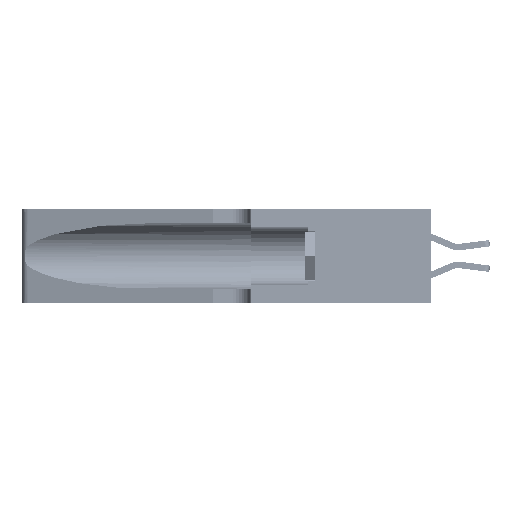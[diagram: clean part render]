
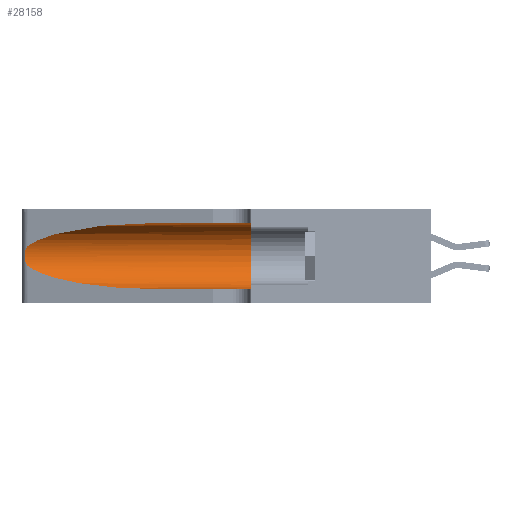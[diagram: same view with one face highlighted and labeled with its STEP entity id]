
A CAD part, left-side view. The second image highlights one B-rep face of the part: STEP entity #28158.
In plain terms, the highlighted cylindrical face has radius 3.308 mm (diameter 6.617 mm), a partial arc.
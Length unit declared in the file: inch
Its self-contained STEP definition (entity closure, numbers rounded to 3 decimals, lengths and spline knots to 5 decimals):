
#955 = EDGE_CURVE ( 'NONE', #9672, #32632, #32036, .T. ) ;
#1538 = DIRECTION ( 'NONE',  ( 0., -1., 0. ) ) ;
#1852 = DIRECTION ( 'NONE',  ( 0., 1., 0. ) ) ;
#2237 = ORIENTED_EDGE ( 'NONE', *, *, #9821, .T. ) ;
#2737 = CARTESIAN_POINT ( 'NONE',  ( 0.25487, 1.22718, 0.22369 ) ) ;
#3219 = CARTESIAN_POINT ( 'NONE',  ( 0.1305, 0.72297, 0.05475 ) ) ;
#3648 = VECTOR ( 'NONE', #16334, 39.37008 ) ;
#4323 = CARTESIAN_POINT ( 'NONE',  ( 0.25487, 1.22718, 0.22369 ) ) ;
#4564 = DIRECTION ( 'NONE',  ( 0., 0., -1. ) ) ;
#4665 = CIRCLE ( 'NONE', #30222, 0.13025 ) ;
#6470 = VERTEX_POINT ( 'NONE', #3219 ) ;
#8814 = CARTESIAN_POINT ( 'NONE',  ( 0.25639, 1.23184, 0.21858 ) ) ;
#9280 = EDGE_CURVE ( 'NONE', #32632, #34541, #4665, .T. ) ;
#9672 = VERTEX_POINT ( 'NONE', #33567 ) ;
#9786 = FACE_OUTER_BOUND ( 'NONE', #30155, .T. ) ;
#9821 = EDGE_CURVE ( 'NONE', #9672, #14651, #11032, .T. ) ;
#10964 = CARTESIAN_POINT ( 'NONE',  ( 0.25789, 1.23486, 0.15765 ) ) ;
#11032 =( BOUNDED_CURVE ( )  B_SPLINE_CURVE ( 3, ( #16282, #19307, #22348, #4323 ),
 .UNSPECIFIED., .F., .F. ) 
 B_SPLINE_CURVE_WITH_KNOTS ( ( 4, 4 ),
 ( 1.5708, 2.84003 ),
 .UNSPECIFIED. ) 
 CURVE ( )  GEOMETRIC_REPRESENTATION_ITEM ( )  RATIONAL_B_SPLINE_CURVE ( ( 1., 0.87, 0.87, 1. ) ) 
 REPRESENTATION_ITEM ( '' )  );
#11691 = CARTESIAN_POINT ( 'NONE',  ( 0.25555, 1.22994, 0.2215 ) ) ;
#11820 = CARTESIAN_POINT ( 'NONE',  ( 0.25854, 1.2359, 0.20912 ) ) ;
#11957 = CARTESIAN_POINT ( 'NONE',  ( 0.2373, 1.15595, 0.08982 ) ) ;
#13049 = EDGE_CURVE ( 'NONE', #14651, #28102, #31943, .T. ) ;
#13907 =( BOUNDED_CURVE ( )  B_SPLINE_CURVE ( 3, ( #14707, #11957, #18015, #24111 ),
 .UNSPECIFIED., .F., .F. ) 
 B_SPLINE_CURVE_WITH_KNOTS ( ( 4, 4 ),
 ( 3.44316, 4.71239 ),
 .UNSPECIFIED. ) 
 CURVE ( )  GEOMETRIC_REPRESENTATION_ITEM ( )  RATIONAL_B_SPLINE_CURVE ( ( 1., 0.87, 0.87, 1. ) ) 
 REPRESENTATION_ITEM ( '' )  );
#13972 = CARTESIAN_POINT ( 'NONE',  ( 0.25555, 1.22993, 0.14849 ) ) ;
#14651 = VERTEX_POINT ( 'NONE', #38706 ) ;
#14707 = CARTESIAN_POINT ( 'NONE',  ( 0.25487, 1.22718, 0.14631 ) ) ;
#14832 = CARTESIAN_POINT ( 'NONE',  ( 0.26075, 1.23896, 0.19203 ) ) ;
#15405 = ORIENTED_EDGE ( 'NONE', *, *, #35889, .T. ) ;
#16178 = CARTESIAN_POINT ( 'NONE',  ( 0.1305, 1.61858, 0.31525 ) ) ;
#16282 = CARTESIAN_POINT ( 'NONE',  ( 0.1305, 0.72297, 0.31525 ) ) ;
#16334 = DIRECTION ( 'NONE',  ( 0., -1., 0. ) ) ;
#16691 = CARTESIAN_POINT ( 'NONE',  ( 0.1305, 0.35, 0.05475 ) ) ;
#17156 = EDGE_CURVE ( 'NONE', #28102, #6470, #13907, .T. ) ;
#17339 = CARTESIAN_POINT ( 'NONE',  ( 0.25856, 1.23593, 0.16098 ) ) ;
#17886 = CARTESIAN_POINT ( 'NONE',  ( 0.26017, 1.23833, 0.17102 ) ) ;
#18015 = CARTESIAN_POINT ( 'NONE',  ( 0.18966, 0.96281, 0.05475 ) ) ;
#19307 = CARTESIAN_POINT ( 'NONE',  ( 0.18966, 0.96281, 0.31525 ) ) ;
#19891 = CARTESIAN_POINT ( 'NONE',  ( 0.1305, 0.35, 0.185 ) ) ;
#22348 = CARTESIAN_POINT ( 'NONE',  ( 0.2373, 1.15595, 0.28018 ) ) ;
#22912 = DIRECTION ( 'NONE',  ( 0., 0., 1. ) ) ;
#24111 = CARTESIAN_POINT ( 'NONE',  ( 0.1305, 0.72297, 0.05475 ) ) ;
#28102 = VERTEX_POINT ( 'NONE', #34190 ) ;
#28158 = ADVANCED_FACE ( 'NONE', ( #9786 ), #31838, .F. ) ;
#28571 = ORIENTED_EDGE ( 'NONE', *, *, #9280, .F. ) ;
#29656 = CARTESIAN_POINT ( 'NONE',  ( 0.1305, 0.35, 0.31525 ) ) ;
#29827 = CARTESIAN_POINT ( 'NONE',  ( 0.25787, 1.23484, 0.2124 ) ) ;
#30155 = EDGE_LOOP ( 'NONE', ( #2237, #36306, #33506, #15405, #28571, #35511 ) ) ;
#30222 = AXIS2_PLACEMENT_3D ( 'NONE', #19891, #1852, #22912 ) ;
#31088 = VECTOR ( 'NONE', #34088, 39.37008 ) ;
#31274 = CARTESIAN_POINT ( 'NONE',  ( 0.1305, 1.61858, 0.05475 ) ) ;
#31838 = CYLINDRICAL_SURFACE ( 'NONE', #34426, 0.13025 ) ;
#31938 = CARTESIAN_POINT ( 'NONE',  ( 0.25639, 1.23186, 0.15144 ) ) ;
#31943 = B_SPLINE_CURVE_WITH_KNOTS ( 'NONE', 3,
 ( #2737, #11691, #8814, #29827, #11820, #32785, #14832, #35764, #17886, #17339, #10964, #31938, #13972, #34893 ),
 .UNSPECIFIED., .F., .F.,
 ( 4, 2, 2, 2, 2, 2, 4 ),
 ( 0., 0.00027, 0.00053, 0.00107, 0.0016, 0.00187, 0.00214 ),
 .UNSPECIFIED. ) ;
#32036 = LINE ( 'NONE', #16178, #31088 ) ;
#32632 = VERTEX_POINT ( 'NONE', #29656 ) ;
#32785 = CARTESIAN_POINT ( 'NONE',  ( 0.26018, 1.23835, 0.19895 ) ) ;
#33506 = ORIENTED_EDGE ( 'NONE', *, *, #17156, .T. ) ;
#33567 = CARTESIAN_POINT ( 'NONE',  ( 0.1305, 0.72297, 0.31525 ) ) ;
#34088 = DIRECTION ( 'NONE',  ( 0., -1., 0. ) ) ;
#34190 = CARTESIAN_POINT ( 'NONE',  ( 0.25487, 1.22718, 0.14631 ) ) ;
#34426 = AXIS2_PLACEMENT_3D ( 'NONE', #34446, #1538, #4564 ) ;
#34446 = CARTESIAN_POINT ( 'NONE',  ( 0.1305, 1.61858, 0.185 ) ) ;
#34541 = VERTEX_POINT ( 'NONE', #16691 ) ;
#34893 = CARTESIAN_POINT ( 'NONE',  ( 0.25487, 1.22718, 0.14631 ) ) ;
#35511 = ORIENTED_EDGE ( 'NONE', *, *, #955, .F. ) ;
#35528 = LINE ( 'NONE', #31274, #3648 ) ;
#35764 = CARTESIAN_POINT ( 'NONE',  ( 0.26075, 1.23896, 0.178 ) ) ;
#35889 = EDGE_CURVE ( 'NONE', #6470, #34541, #35528, .T. ) ;
#36306 = ORIENTED_EDGE ( 'NONE', *, *, #13049, .T. ) ;
#38706 = CARTESIAN_POINT ( 'NONE',  ( 0.25487, 1.22718, 0.22369 ) ) ;
